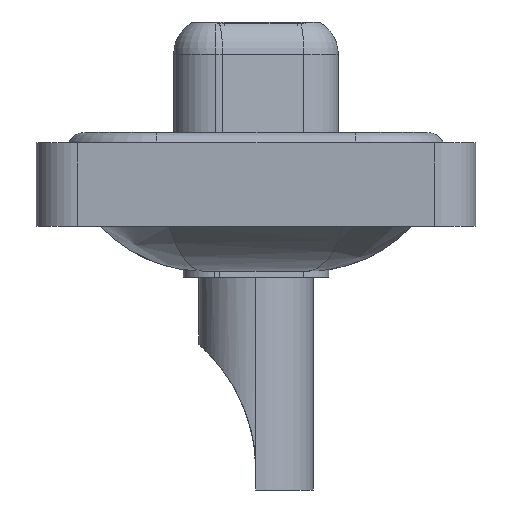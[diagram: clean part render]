
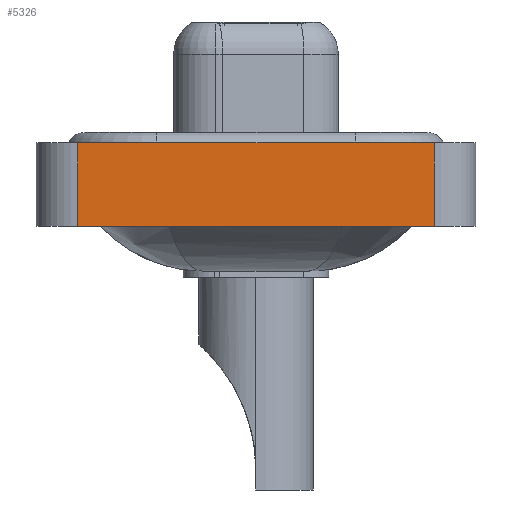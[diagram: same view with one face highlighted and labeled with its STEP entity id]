
A CAD part, left-side view. The second image highlights one B-rep face of the part: STEP entity #5326.
In plain terms, the highlighted planar face has unit normal (-1, 0, 0).
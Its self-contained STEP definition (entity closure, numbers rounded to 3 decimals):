
#170 = ORIENTED_EDGE ( 'NONE', *, *, #6467, .T. ) ;
#457 = DIRECTION ( 'NONE',  ( 0., -1., 0. ) ) ;
#567 = LINE ( 'NONE', #3307, #6385 ) ;
#1035 = LINE ( 'NONE', #11679, #15870 ) ;
#1099 = CARTESIAN_POINT ( 'NONE',  ( -7.3, -8.55, -3.6 ) ) ;
#1255 = CARTESIAN_POINT ( 'NONE',  ( -7.3, -8.55, -3.6 ) ) ;
#2505 = LINE ( 'NONE', #1099, #12309 ) ;
#2556 = CARTESIAN_POINT ( 'NONE',  ( -7.3, -8.55, 0.4 ) ) ;
#2559 = DIRECTION ( 'NONE',  ( 0., 0., 1. ) ) ;
#3096 = CARTESIAN_POINT ( 'NONE',  ( -7.3, -8.55, -3.6 ) ) ;
#3297 = VERTEX_POINT ( 'NONE', #4892 ) ;
#3307 = CARTESIAN_POINT ( 'NONE',  ( -7.3, 8.55, -3.6 ) ) ;
#3729 = AXIS2_PLACEMENT_3D ( 'NONE', #9306, #14720, #2559 ) ;
#3855 = ORIENTED_EDGE ( 'NONE', *, *, #14796, .F. ) ;
#3898 = PLANE ( 'NONE',  #3729 ) ;
#4615 = LINE ( 'NONE', #3096, #6247 ) ;
#4892 = CARTESIAN_POINT ( 'NONE',  ( -7.3, 8.55, 0.4 ) ) ;
#4912 = DIRECTION ( 'NONE',  ( 0., 0., 1. ) ) ;
#5269 = VERTEX_POINT ( 'NONE', #1255 ) ;
#5326 = ADVANCED_FACE ( 'NONE', ( #16058 ), #3898, .T. ) ;
#6247 = VECTOR ( 'NONE', #457, 1000. ) ;
#6385 = VECTOR ( 'NONE', #13879, 1000. ) ;
#6467 = EDGE_CURVE ( 'NONE', #10468, #5269, #4615, .T. ) ;
#8991 = DIRECTION ( 'NONE',  ( 0., -1., 0. ) ) ;
#9088 = EDGE_CURVE ( 'NONE', #3297, #15277, #1035, .T. ) ;
#9306 = CARTESIAN_POINT ( 'NONE',  ( -7.3, -8.55, -3.6 ) ) ;
#9686 = CARTESIAN_POINT ( 'NONE',  ( -7.3, 8.55, -3.6 ) ) ;
#10468 = VERTEX_POINT ( 'NONE', #9686 ) ;
#11189 = ORIENTED_EDGE ( 'NONE', *, *, #13268, .T. ) ;
#11679 = CARTESIAN_POINT ( 'NONE',  ( -7.3, -8.55, 0.4 ) ) ;
#12309 = VECTOR ( 'NONE', #4912, 1000. ) ;
#13268 = EDGE_CURVE ( 'NONE', #5269, #15277, #2505, .T. ) ;
#13879 = DIRECTION ( 'NONE',  ( 0., 0., 1. ) ) ;
#14720 = DIRECTION ( 'NONE',  ( -1., 0., 0. ) ) ;
#14796 = EDGE_CURVE ( 'NONE', #10468, #3297, #567, .T. ) ;
#15277 = VERTEX_POINT ( 'NONE', #2556 ) ;
#15870 = VECTOR ( 'NONE', #8991, 1000. ) ;
#16058 = FACE_OUTER_BOUND ( 'NONE', #16472, .T. ) ;
#16472 = EDGE_LOOP ( 'NONE', ( #11189, #16616, #3855, #170 ) ) ;
#16616 = ORIENTED_EDGE ( 'NONE', *, *, #9088, .F. ) ;
